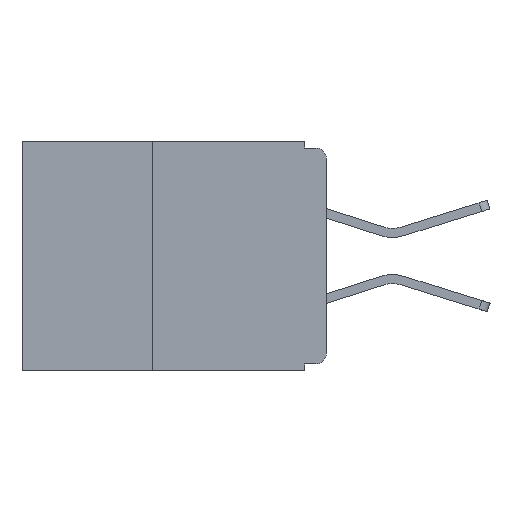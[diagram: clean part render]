
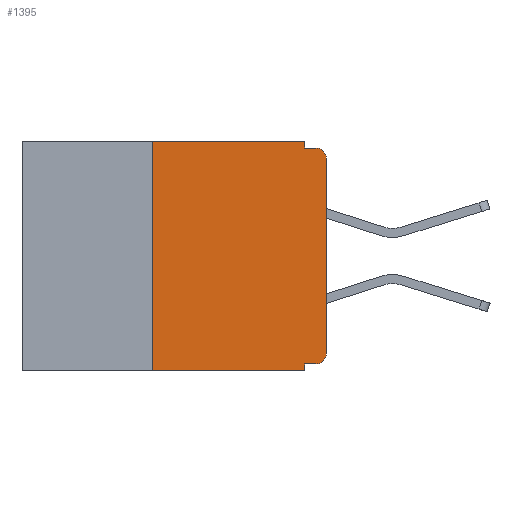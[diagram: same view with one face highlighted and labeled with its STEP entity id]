
A CAD part, left-side view. The second image highlights one B-rep face of the part: STEP entity #1395.
In plain terms, the highlighted planar face has unit normal (-1, 0, 0).
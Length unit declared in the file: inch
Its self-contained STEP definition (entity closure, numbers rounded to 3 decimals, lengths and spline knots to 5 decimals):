
#238 = VERTEX_POINT ( 'NONE', #6971 ) ;
#468 = VERTEX_POINT ( 'NONE', #2878 ) ;
#544 = VERTEX_POINT ( 'NONE', #5264 ) ;
#557 = CARTESIAN_POINT ( 'NONE',  ( 0., 0., 0. ) ) ;
#561 = DIRECTION ( 'NONE',  ( 0., 0., -1. ) ) ;
#605 = ORIENTED_EDGE ( 'NONE', *, *, #1369, .F. ) ;
#960 = AXIS2_PLACEMENT_3D ( 'NONE', #5167, #13391, #6419 ) ;
#965 = DIRECTION ( 'NONE',  ( 0., -1., 0. ) ) ;
#1035 = LINE ( 'NONE', #6770, #10325 ) ;
#1213 = VECTOR ( 'NONE', #11838, 39.37008 ) ;
#1369 = EDGE_CURVE ( 'NONE', #3002, #2322, #8800, .T. ) ;
#1395 = ADVANCED_FACE ( 'NONE', ( #7713 ), #7775, .F. ) ;
#1416 = CARTESIAN_POINT ( 'NONE',  ( 0., 0., -0.01 ) ) ;
#1539 = CARTESIAN_POINT ( 'NONE',  ( 0., 0., -0.025 ) ) ;
#1744 = ORIENTED_EDGE ( 'NONE', *, *, #11928, .T. ) ;
#2322 = VERTEX_POINT ( 'NONE', #12798 ) ;
#2332 = CARTESIAN_POINT ( 'NONE',  ( 0., 0.437, 0. ) ) ;
#2694 = VERTEX_POINT ( 'NONE', #8072 ) ;
#2741 = VERTEX_POINT ( 'NONE', #8235 ) ;
#2859 = LINE ( 'NONE', #6305, #12064 ) ;
#2878 = CARTESIAN_POINT ( 'NONE',  ( 0., 0.031, -0.33 ) ) ;
#2930 = AXIS2_PLACEMENT_3D ( 'NONE', #4572, #4542, #4524 ) ;
#3002 = VERTEX_POINT ( 'NONE', #3748 ) ;
#3010 = AXIS2_PLACEMENT_3D ( 'NONE', #3689, #7759, #7747 ) ;
#3276 = LINE ( 'NONE', #1416, #5859 ) ;
#3361 = CARTESIAN_POINT ( 'NONE',  ( 0., 0., -0.32 ) ) ;
#3496 = DIRECTION ( 'NONE',  ( 0., 1., 0. ) ) ;
#3689 = CARTESIAN_POINT ( 'NONE',  ( 0., 0.437, 0. ) ) ;
#3716 = VERTEX_POINT ( 'NONE', #1539 ) ;
#3748 = CARTESIAN_POINT ( 'NONE',  ( 0., 0.015, -0.32 ) ) ;
#4207 = VECTOR ( 'NONE', #15415, 39.37008 ) ;
#4226 = CARTESIAN_POINT ( 'NONE',  ( 0., 0.031, 0. ) ) ;
#4524 = DIRECTION ( 'NONE',  ( 0., 0., -1. ) ) ;
#4542 = DIRECTION ( 'NONE',  ( -1., 0., 0. ) ) ;
#4572 = CARTESIAN_POINT ( 'NONE',  ( 0., 0.015, -0.305 ) ) ;
#5167 = CARTESIAN_POINT ( 'NONE',  ( 0., 0.015, -0.025 ) ) ;
#5249 = LINE ( 'NONE', #4226, #11215 ) ;
#5264 = CARTESIAN_POINT ( 'NONE',  ( 0., 0.015, -0.01 ) ) ;
#5608 = LINE ( 'NONE', #557, #8420 ) ;
#5749 = ORIENTED_EDGE ( 'NONE', *, *, #13387, .T. ) ;
#5859 = VECTOR ( 'NONE', #965, 39.37008 ) ;
#6199 = DIRECTION ( 'NONE',  ( 0., 0., -1. ) ) ;
#6288 = CARTESIAN_POINT ( 'NONE',  ( 0., 0.031, -0.01 ) ) ;
#6305 = CARTESIAN_POINT ( 'NONE',  ( 0., 0.031, -0.33 ) ) ;
#6419 = DIRECTION ( 'NONE',  ( 0., 0., -1. ) ) ;
#6684 = DIRECTION ( 'NONE',  ( 0., 0., 1. ) ) ;
#6756 = EDGE_LOOP ( 'NONE', ( #10886, #5749, #8192, #10126, #11599, #9412, #7403, #13212, #605, #1744 ) ) ;
#6770 = CARTESIAN_POINT ( 'NONE',  ( 0., 0.25, -0.33 ) ) ;
#6823 = EDGE_CURVE ( 'NONE', #2694, #468, #7782, .T. ) ;
#6971 = CARTESIAN_POINT ( 'NONE',  ( 0., 0.031, 0. ) ) ;
#7067 = CARTESIAN_POINT ( 'NONE',  ( 0., 0.25, 0. ) ) ;
#7093 = EDGE_CURVE ( 'NONE', #2694, #9672, #1035, .T. ) ;
#7403 = ORIENTED_EDGE ( 'NONE', *, *, #6823, .T. ) ;
#7490 = LINE ( 'NONE', #2332, #4207 ) ;
#7713 = FACE_OUTER_BOUND ( 'NONE', #6756, .T. ) ;
#7747 = DIRECTION ( 'NONE',  ( 0., 0., -1. ) ) ;
#7759 = DIRECTION ( 'NONE',  ( 1., 0., 0. ) ) ;
#7775 = PLANE ( 'NONE',  #3010 ) ;
#7782 = LINE ( 'NONE', #11816, #1213 ) ;
#8072 = CARTESIAN_POINT ( 'NONE',  ( 0., 0.25, -0.33 ) ) ;
#8192 = ORIENTED_EDGE ( 'NONE', *, *, #12080, .F. ) ;
#8235 = CARTESIAN_POINT ( 'NONE',  ( 0., 0., -0.305 ) ) ;
#8420 = VECTOR ( 'NONE', #10275, 39.37008 ) ;
#8665 = EDGE_CURVE ( 'NONE', #2322, #468, #2859, .T. ) ;
#8800 = LINE ( 'NONE', #3361, #13832 ) ;
#9412 = ORIENTED_EDGE ( 'NONE', *, *, #7093, .F. ) ;
#9672 = VERTEX_POINT ( 'NONE', #7067 ) ;
#10126 = ORIENTED_EDGE ( 'NONE', *, *, #12346, .F. ) ;
#10275 = DIRECTION ( 'NONE',  ( 0., 0., 1. ) ) ;
#10325 = VECTOR ( 'NONE', #6684, 39.37008 ) ;
#10886 = ORIENTED_EDGE ( 'NONE', *, *, #14168, .T. ) ;
#11215 = VECTOR ( 'NONE', #561, 39.37008 ) ;
#11599 = ORIENTED_EDGE ( 'NONE', *, *, #14930, .F. ) ;
#11816 = CARTESIAN_POINT ( 'NONE',  ( 0., 0.437, -0.33 ) ) ;
#11838 = DIRECTION ( 'NONE',  ( 0., -1., 0. ) ) ;
#11928 = EDGE_CURVE ( 'NONE', #3002, #2741, #14244, .T. ) ;
#12064 = VECTOR ( 'NONE', #6199, 39.37008 ) ;
#12080 = EDGE_CURVE ( 'NONE', #12169, #544, #3276, .T. ) ;
#12169 = VERTEX_POINT ( 'NONE', #6288 ) ;
#12346 = EDGE_CURVE ( 'NONE', #238, #12169, #5249, .T. ) ;
#12798 = CARTESIAN_POINT ( 'NONE',  ( 0., 0.031, -0.32 ) ) ;
#13212 = ORIENTED_EDGE ( 'NONE', *, *, #8665, .F. ) ;
#13387 = EDGE_CURVE ( 'NONE', #3716, #544, #14585, .T. ) ;
#13391 = DIRECTION ( 'NONE',  ( -1., 0., 0. ) ) ;
#13832 = VECTOR ( 'NONE', #3496, 39.37008 ) ;
#14168 = EDGE_CURVE ( 'NONE', #2741, #3716, #5608, .T. ) ;
#14244 = CIRCLE ( 'NONE', #2930, 0.015 ) ;
#14585 = CIRCLE ( 'NONE', #960, 0.015 ) ;
#14930 = EDGE_CURVE ( 'NONE', #9672, #238, #7490, .T. ) ;
#15415 = DIRECTION ( 'NONE',  ( 0., -1., 0. ) ) ;
